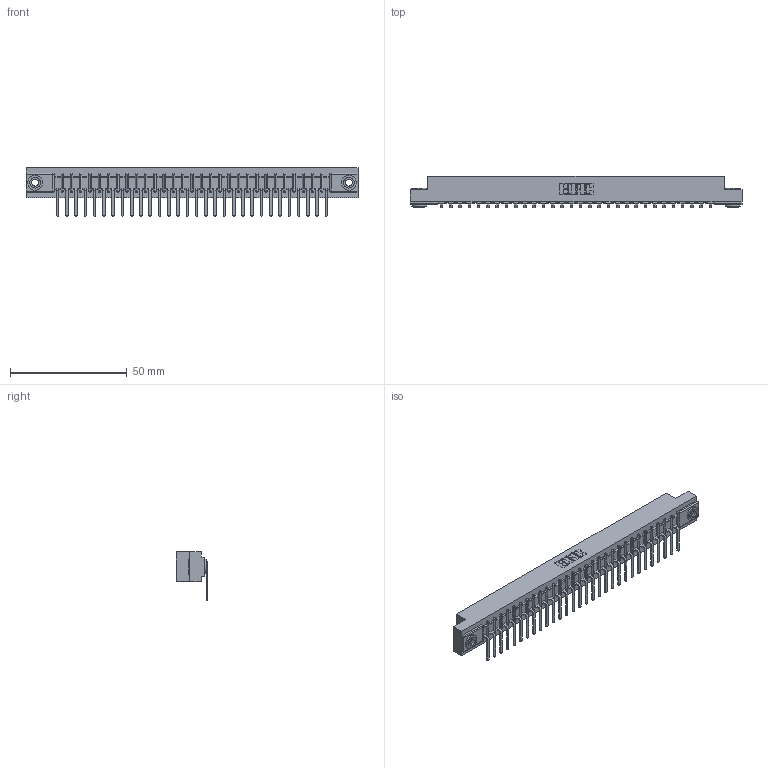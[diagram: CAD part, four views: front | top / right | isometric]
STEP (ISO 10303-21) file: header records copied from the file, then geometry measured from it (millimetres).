
FILE_DESCRIPTION (( 'STEP AP203' ), '1' );
FILE_NAME ('357-030-557-103.STEP', '2018-08-09T09:37:36', ( '' ), ( '' ), 'SwSTEP 2.0', 'SolidWorks 2016', '' );
FILE_SCHEMA (( 'CONFIG_CONTROL_DESIGN' ));
Length unit declared in the file: inch
Products named in the file (4): 307-290-002_557; 345-250-002_345-250-002-102; 357-030-557-103; 307 Part_.156 Dia Mounting Holes
Assembly tree (33 placements, depth 2):
  357-030-557-103
    307 Part_.156 Dia Mounting Holes
    307-290-002_557  x30
    345-250-002_345-250-002-102  x2
Bounding box: 141.88 x 13.36 x 20.66 mm (x, y, z)
Volume: 15176.2 mm3; surface area: 19594.7 mm2
Topology: 33 solids, 33 shells, 2541 faces, 7755 edges, 5082 vertices
Faces by surface type: plane 1504, cylinder 967, sphere 62, cone 8
Entity records: 29117 total; most frequent: CARTESIAN_POINT 4889, ORIENTED_EDGE 4870, DIRECTION 4771, EDGE_CURVE 2435, LINE 1851, VECTOR 1851, VERTEX_POINT 1578, AXIS2_PLACEMENT_3D 1460
